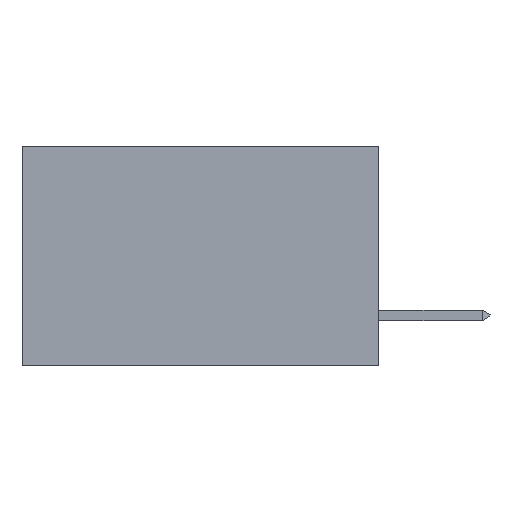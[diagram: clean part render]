
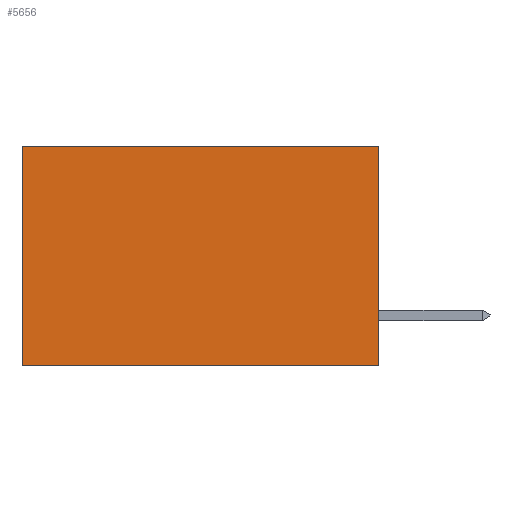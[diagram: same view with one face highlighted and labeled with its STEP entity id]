
A CAD part, left-side view. The second image highlights one B-rep face of the part: STEP entity #5656.
In plain terms, the highlighted planar face has unit normal (-1, 0, 0).
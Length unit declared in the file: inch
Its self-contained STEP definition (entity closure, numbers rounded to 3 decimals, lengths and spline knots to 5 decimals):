
#63 = VECTOR ( 'NONE', #10286, 39.37008 ) ;
#923 = VERTEX_POINT ( 'NONE', #5209 ) ;
#2655 = DIRECTION ( 'NONE',  ( 0., 0., -1. ) ) ;
#2933 = LINE ( 'NONE', #6374, #3837 ) ;
#3729 = CARTESIAN_POINT ( 'NONE',  ( 0.2615, 0.6, 0. ) ) ;
#3837 = VECTOR ( 'NONE', #13740, 39.37008 ) ;
#4211 = ORIENTED_EDGE ( 'NONE', *, *, #8699, .T. ) ;
#4547 = DIRECTION ( 'NONE',  ( 0., 1., 0. ) ) ;
#5209 = CARTESIAN_POINT ( 'NONE',  ( 0.2615, 0., -0.37 ) ) ;
#5656 = ADVANCED_FACE ( 'NONE', ( #8675 ), #13354, .F. ) ;
#5814 = DIRECTION ( 'NONE',  ( 0., 0., -1. ) ) ;
#6060 = CARTESIAN_POINT ( 'NONE',  ( 0.2615, 0., -0.37 ) ) ;
#6335 = VERTEX_POINT ( 'NONE', #9671 ) ;
#6374 = CARTESIAN_POINT ( 'NONE',  ( 0.2615, 0., 0. ) ) ;
#6415 = ORIENTED_EDGE ( 'NONE', *, *, #12623, .F. ) ;
#7149 = AXIS2_PLACEMENT_3D ( 'NONE', #11938, #10404, #2655 ) ;
#7552 = VERTEX_POINT ( 'NONE', #3729 ) ;
#8675 = FACE_OUTER_BOUND ( 'NONE', #17311, .T. ) ;
#8692 = CARTESIAN_POINT ( 'NONE',  ( 0.2615, 0.6, -0.37 ) ) ;
#8699 = EDGE_CURVE ( 'NONE', #19094, #7552, #2933, .T. ) ;
#9145 = LINE ( 'NONE', #6060, #12788 ) ;
#9671 = CARTESIAN_POINT ( 'NONE',  ( 0.2615, 0.6, -0.37 ) ) ;
#9752 = ORIENTED_EDGE ( 'NONE', *, *, #18272, .T. ) ;
#10286 = DIRECTION ( 'NONE',  ( 0., 0., -1. ) ) ;
#10318 = LINE ( 'NONE', #8692, #19145 ) ;
#10404 = DIRECTION ( 'NONE',  ( 1., 0., 0. ) ) ;
#11938 = CARTESIAN_POINT ( 'NONE',  ( 0.2615, 0., -0.37 ) ) ;
#12396 = CARTESIAN_POINT ( 'NONE',  ( 0.2615, 0., 0. ) ) ;
#12623 = EDGE_CURVE ( 'NONE', #19094, #923, #18063, .T. ) ;
#12788 = VECTOR ( 'NONE', #4547, 39.37008 ) ;
#13205 = EDGE_CURVE ( 'NONE', #923, #6335, #9145, .T. ) ;
#13354 = PLANE ( 'NONE',  #7149 ) ;
#13740 = DIRECTION ( 'NONE',  ( 0., 1., 0. ) ) ;
#16227 = CARTESIAN_POINT ( 'NONE',  ( 0.2615, 0., -0.37 ) ) ;
#16309 = ORIENTED_EDGE ( 'NONE', *, *, #13205, .F. ) ;
#17311 = EDGE_LOOP ( 'NONE', ( #9752, #16309, #6415, #4211 ) ) ;
#18063 = LINE ( 'NONE', #16227, #63 ) ;
#18272 = EDGE_CURVE ( 'NONE', #7552, #6335, #10318, .T. ) ;
#19094 = VERTEX_POINT ( 'NONE', #12396 ) ;
#19145 = VECTOR ( 'NONE', #5814, 39.37008 ) ;
